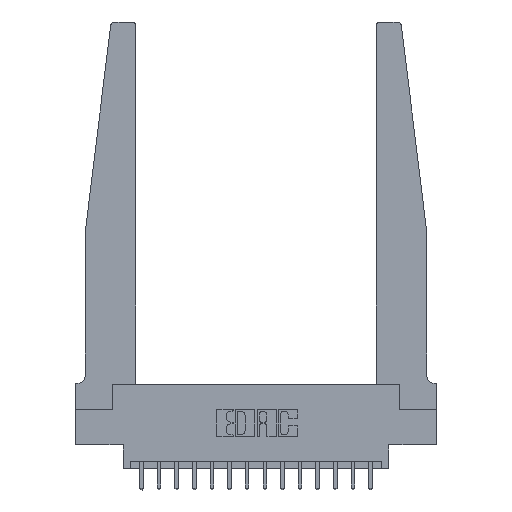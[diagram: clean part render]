
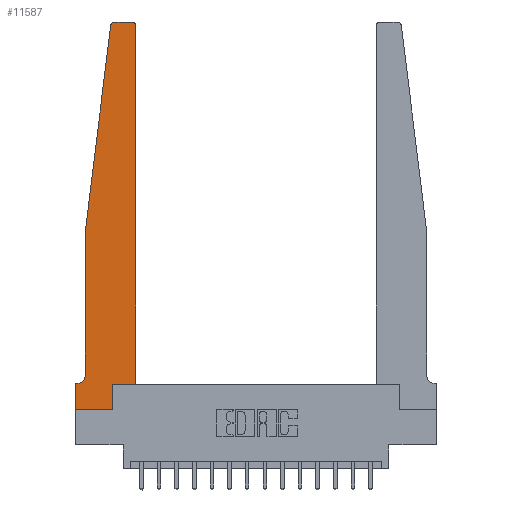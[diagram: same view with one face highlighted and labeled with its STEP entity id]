
A CAD part, top view. The second image highlights one B-rep face of the part: STEP entity #11587.
In plain terms, the highlighted planar face has unit normal (0, 0, 1).
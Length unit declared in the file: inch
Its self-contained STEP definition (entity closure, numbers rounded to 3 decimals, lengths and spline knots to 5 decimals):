
#107 = CARTESIAN_POINT ( 'NONE',  ( 0.065, 0.2375, 0.37 ) ) ;
#213 = ORIENTED_EDGE ( 'NONE', *, *, #13729, .T. ) ;
#593 = VECTOR ( 'NONE', #2318, 39.37008 ) ;
#648 = DIRECTION ( 'NONE',  ( -1., 0., 0. ) ) ;
#901 = ORIENTED_EDGE ( 'NONE', *, *, #13531, .T. ) ;
#974 = PLANE ( 'NONE',  #12955 ) ;
#1270 = DIRECTION ( 'NONE',  ( 0., -1., 0. ) ) ;
#1517 = CARTESIAN_POINT ( 'NONE',  ( 0.27653, 2.72, 0.37 ) ) ;
#1519 = FACE_OUTER_BOUND ( 'NONE', #3801, .T. ) ;
#1711 = CARTESIAN_POINT ( 'NONE',  ( 0., 0., 0.37 ) ) ;
#1751 = CARTESIAN_POINT ( 'NONE',  ( 0.015, 0.2375, 0.37 ) ) ;
#1888 = LINE ( 'NONE', #8093, #5208 ) ;
#1997 = ORIENTED_EDGE ( 'NONE', *, *, #17217, .T. ) ;
#2318 = DIRECTION ( 'NONE',  ( 0., -1., 0. ) ) ;
#2395 = CARTESIAN_POINT ( 'NONE',  ( 0., 0.1875, 0.37 ) ) ;
#2565 = DIRECTION ( 'NONE',  ( 1., 0., 0. ) ) ;
#2795 = CIRCLE ( 'NONE', #11063, 0.05 ) ;
#2936 = DIRECTION ( 'NONE',  ( 1., 0., 0. ) ) ;
#3146 = VERTEX_POINT ( 'NONE', #107 ) ;
#3162 = EDGE_CURVE ( 'NONE', #14275, #4692, #10372, .T. ) ;
#3170 = DIRECTION ( 'NONE',  ( -1., 0., 0. ) ) ;
#3404 = VECTOR ( 'NONE', #6568, 39.37008 ) ;
#3556 = EDGE_CURVE ( 'NONE', #4157, #7376, #11665, .T. ) ;
#3636 = VERTEX_POINT ( 'NONE', #12105 ) ;
#3651 = CARTESIAN_POINT ( 'NONE',  ( 0.24675, 2.72367, 0.37 ) ) ;
#3746 = CARTESIAN_POINT ( 'NONE',  ( 0.395, 2.72, 0.37 ) ) ;
#3786 = AXIS2_PLACEMENT_3D ( 'NONE', #3746, #13361, #5190 ) ;
#3801 = EDGE_LOOP ( 'NONE', ( #16641, #213, #6155, #1997, #9017, #13696, #16675, #901, #3899, #17295, #14720, #6231 ) ) ;
#3899 = ORIENTED_EDGE ( 'NONE', *, *, #3162, .T. ) ;
#3916 = VERTEX_POINT ( 'NONE', #7467 ) ;
#4157 = VERTEX_POINT ( 'NONE', #6685 ) ;
#4692 = VERTEX_POINT ( 'NONE', #14554 ) ;
#4925 = CARTESIAN_POINT ( 'NONE',  ( 0.065, 0.1875, 0.37 ) ) ;
#5115 = CARTESIAN_POINT ( 'NONE',  ( 0., 0., 0.37 ) ) ;
#5163 = CIRCLE ( 'NONE', #9873, 0.03 ) ;
#5176 = VECTOR ( 'NONE', #17162, 39.37008 ) ;
#5190 = DIRECTION ( 'NONE',  ( 1., 0., 0. ) ) ;
#5208 = VECTOR ( 'NONE', #2565, 39.37008 ) ;
#5253 = DIRECTION ( 'NONE',  ( 0., 0., 1. ) ) ;
#5782 = DIRECTION ( 'NONE',  ( 0., 1., 0. ) ) ;
#6155 = ORIENTED_EDGE ( 'NONE', *, *, #6550, .T. ) ;
#6215 = EDGE_CURVE ( 'NONE', #3146, #10443, #2795, .T. ) ;
#6231 = ORIENTED_EDGE ( 'NONE', *, *, #15250, .T. ) ;
#6481 = VERTEX_POINT ( 'NONE', #3651 ) ;
#6550 = EDGE_CURVE ( 'NONE', #6481, #10376, #11866, .T. ) ;
#6568 = DIRECTION ( 'NONE',  ( -1., 0., 0. ) ) ;
#6571 = VERTEX_POINT ( 'NONE', #12082 ) ;
#6685 = CARTESIAN_POINT ( 'NONE',  ( 0., 0.1875, 0.37 ) ) ;
#6961 = DIRECTION ( 'NONE',  ( 1., 0., 0. ) ) ;
#7373 = VECTOR ( 'NONE', #1270, 39.37008 ) ;
#7376 = VERTEX_POINT ( 'NONE', #1711 ) ;
#7467 = CARTESIAN_POINT ( 'NONE',  ( 0.27653, 2.75, 0.37 ) ) ;
#7598 = EDGE_CURVE ( 'NONE', #10443, #4157, #15427, .T. ) ;
#7750 = VECTOR ( 'NONE', #648, 39.37008 ) ;
#7903 = VERTEX_POINT ( 'NONE', #10100 ) ;
#8093 = CARTESIAN_POINT ( 'NONE',  ( 0.425, 0.18, 0.37 ) ) ;
#8152 = LINE ( 'NONE', #13771, #14551 ) ;
#8224 = CARTESIAN_POINT ( 'NONE',  ( 0.065, 1.25, 0.37 ) ) ;
#8645 = VECTOR ( 'NONE', #16103, 39.37008 ) ;
#9017 = ORIENTED_EDGE ( 'NONE', *, *, #6215, .T. ) ;
#9520 = CARTESIAN_POINT ( 'NONE',  ( 0.065, 1.25, 0.37 ) ) ;
#9691 = CARTESIAN_POINT ( 'NONE',  ( 0.015, 0.1875, 0.37 ) ) ;
#9873 = AXIS2_PLACEMENT_3D ( 'NONE', #1517, #11208, #2936 ) ;
#9939 = VECTOR ( 'NONE', #5782, 39.37008 ) ;
#10100 = CARTESIAN_POINT ( 'NONE',  ( 0.425, 0.18, 0.37 ) ) ;
#10372 = LINE ( 'NONE', #15314, #9939 ) ;
#10376 = VERTEX_POINT ( 'NONE', #9520 ) ;
#10384 = CARTESIAN_POINT ( 'NONE',  ( 0.425, 0.18, 0.37 ) ) ;
#10443 = VERTEX_POINT ( 'NONE', #9691 ) ;
#10647 = CIRCLE ( 'NONE', #3786, 0.03 ) ;
#11063 = AXIS2_PLACEMENT_3D ( 'NONE', #1751, #11433, #3170 ) ;
#11170 = LINE ( 'NONE', #16102, #3404 ) ;
#11208 = DIRECTION ( 'NONE',  ( 0., 0., 1. ) ) ;
#11433 = DIRECTION ( 'NONE',  ( 0., 0., -1. ) ) ;
#11587 = ADVANCED_FACE ( 'NONE', ( #1519 ), #974, .T. ) ;
#11665 = LINE ( 'NONE', #5115, #593 ) ;
#11866 = LINE ( 'NONE', #14752, #8645 ) ;
#12082 = CARTESIAN_POINT ( 'NONE',  ( 0.425, 2.72, 0.37 ) ) ;
#12105 = CARTESIAN_POINT ( 'NONE',  ( 0.395, 2.75, 0.37 ) ) ;
#12252 = EDGE_CURVE ( 'NONE', #4692, #7903, #1888, .T. ) ;
#12883 = LINE ( 'NONE', #10384, #5176 ) ;
#12904 = EDGE_CURVE ( 'NONE', #3636, #3916, #11170, .T. ) ;
#12955 = AXIS2_PLACEMENT_3D ( 'NONE', #2395, #5253, #14795 ) ;
#13269 = EDGE_CURVE ( 'NONE', #7903, #6571, #12883, .T. ) ;
#13361 = DIRECTION ( 'NONE',  ( 0., 0., 1. ) ) ;
#13531 = EDGE_CURVE ( 'NONE', #7376, #14275, #8152, .T. ) ;
#13696 = ORIENTED_EDGE ( 'NONE', *, *, #7598, .T. ) ;
#13729 = EDGE_CURVE ( 'NONE', #3916, #6481, #5163, .T. ) ;
#13771 = CARTESIAN_POINT ( 'NONE',  ( 0., 0., 0.37 ) ) ;
#14221 = LINE ( 'NONE', #8224, #7373 ) ;
#14275 = VERTEX_POINT ( 'NONE', #14822 ) ;
#14551 = VECTOR ( 'NONE', #6961, 39.37008 ) ;
#14554 = CARTESIAN_POINT ( 'NONE',  ( 0.2605, 0.18, 0.37 ) ) ;
#14720 = ORIENTED_EDGE ( 'NONE', *, *, #13269, .T. ) ;
#14752 = CARTESIAN_POINT ( 'NONE',  ( 0.065, 1.25, 0.37 ) ) ;
#14795 = DIRECTION ( 'NONE',  ( 1., 0., 0. ) ) ;
#14822 = CARTESIAN_POINT ( 'NONE',  ( 0.2605, 0., 0.37 ) ) ;
#15250 = EDGE_CURVE ( 'NONE', #6571, #3636, #10647, .T. ) ;
#15314 = CARTESIAN_POINT ( 'NONE',  ( 0.2605, 0.18, 0.37 ) ) ;
#15427 = LINE ( 'NONE', #4925, #7750 ) ;
#16102 = CARTESIAN_POINT ( 'NONE',  ( 0.25, 2.75, 0.37 ) ) ;
#16103 = DIRECTION ( 'NONE',  ( -0.122, -0.992, 0. ) ) ;
#16641 = ORIENTED_EDGE ( 'NONE', *, *, #12904, .T. ) ;
#16675 = ORIENTED_EDGE ( 'NONE', *, *, #3556, .T. ) ;
#17162 = DIRECTION ( 'NONE',  ( 0., 1., 0. ) ) ;
#17217 = EDGE_CURVE ( 'NONE', #10376, #3146, #14221, .T. ) ;
#17295 = ORIENTED_EDGE ( 'NONE', *, *, #12252, .T. ) ;
